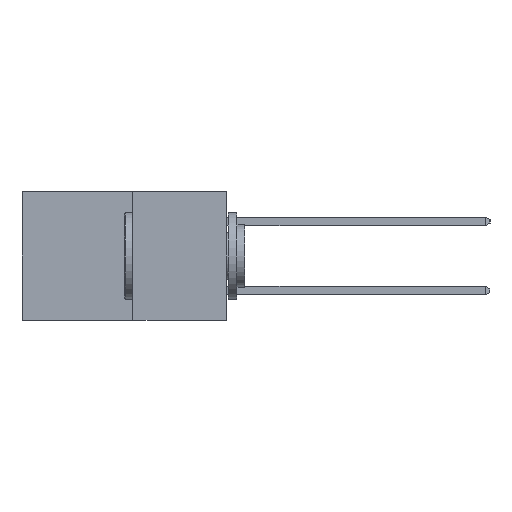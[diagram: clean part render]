
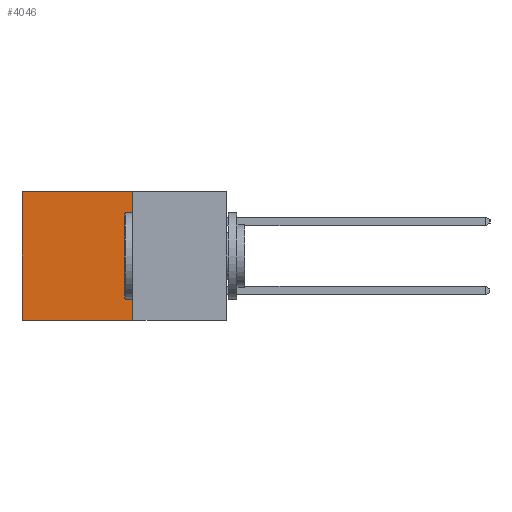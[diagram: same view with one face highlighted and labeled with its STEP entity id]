
A CAD part, left-side view. The second image highlights one B-rep face of the part: STEP entity #4046.
In plain terms, the highlighted planar face has unit normal (-1, 0, 0).
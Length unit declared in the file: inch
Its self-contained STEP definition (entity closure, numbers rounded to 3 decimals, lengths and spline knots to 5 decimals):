
#56 = CARTESIAN_POINT ( 'NONE',  ( 0.277, 0.27, 0. ) ) ;
#151 = DIRECTION ( 'NONE',  ( 0., 1., 0. ) ) ;
#939 = DIRECTION ( 'NONE',  ( 0., 1., 0. ) ) ;
#1374 = EDGE_LOOP ( 'NONE', ( #12339, #5086, #3545, #4096 ) ) ;
#1396 = VERTEX_POINT ( 'NONE', #2069 ) ;
#2069 = CARTESIAN_POINT ( 'NONE',  ( 0.277, 0.59, 0. ) ) ;
#3019 = LINE ( 'NONE', #8699, #11359 ) ;
#3280 = LINE ( 'NONE', #11072, #6197 ) ;
#3545 = ORIENTED_EDGE ( 'NONE', *, *, #8862, .F. ) ;
#3640 = DIRECTION ( 'NONE',  ( 0., 0., -1. ) ) ;
#3840 = EDGE_CURVE ( 'NONE', #12850, #1396, #9208, .T. ) ;
#4020 = CARTESIAN_POINT ( 'NONE',  ( 0.277, 0.59, -0.37 ) ) ;
#4046 = ADVANCED_FACE ( 'NONE', ( #8193 ), #5207, .F. ) ;
#4072 = DIRECTION ( 'NONE',  ( 1., 0., 0. ) ) ;
#4096 = ORIENTED_EDGE ( 'NONE', *, *, #3840, .T. ) ;
#4460 = CARTESIAN_POINT ( 'NONE',  ( 0.277, 0.27, -0.37 ) ) ;
#4951 = EDGE_CURVE ( 'NONE', #7579, #5447, #3019, .T. ) ;
#5086 = ORIENTED_EDGE ( 'NONE', *, *, #4951, .F. ) ;
#5166 = EDGE_CURVE ( 'NONE', #1396, #5447, #13987, .T. ) ;
#5207 = PLANE ( 'NONE',  #6167 ) ;
#5447 = VERTEX_POINT ( 'NONE', #4020 ) ;
#6167 = AXIS2_PLACEMENT_3D ( 'NONE', #4460, #4072, #3640 ) ;
#6197 = VECTOR ( 'NONE', #8925, 39.37008 ) ;
#6520 = DIRECTION ( 'NONE',  ( 0., 0., -1. ) ) ;
#6721 = CARTESIAN_POINT ( 'NONE',  ( 0.277, 0.59, -0.37 ) ) ;
#7237 = CARTESIAN_POINT ( 'NONE',  ( 0.277, 0.27, -0.37 ) ) ;
#7579 = VERTEX_POINT ( 'NONE', #7237 ) ;
#7694 = CARTESIAN_POINT ( 'NONE',  ( 0.277, 0.27, 0. ) ) ;
#8193 = FACE_OUTER_BOUND ( 'NONE', #1374, .T. ) ;
#8699 = CARTESIAN_POINT ( 'NONE',  ( 0.277, 0.27, -0.37 ) ) ;
#8862 = EDGE_CURVE ( 'NONE', #12850, #7579, #3280, .T. ) ;
#8866 = VECTOR ( 'NONE', #151, 39.37008 ) ;
#8925 = DIRECTION ( 'NONE',  ( 0., 0., -1. ) ) ;
#9208 = LINE ( 'NONE', #56, #8866 ) ;
#11072 = CARTESIAN_POINT ( 'NONE',  ( 0.277, 0.27, -0.37 ) ) ;
#11176 = VECTOR ( 'NONE', #6520, 39.37008 ) ;
#11359 = VECTOR ( 'NONE', #939, 39.37008 ) ;
#12339 = ORIENTED_EDGE ( 'NONE', *, *, #5166, .T. ) ;
#12850 = VERTEX_POINT ( 'NONE', #7694 ) ;
#13987 = LINE ( 'NONE', #6721, #11176 ) ;
